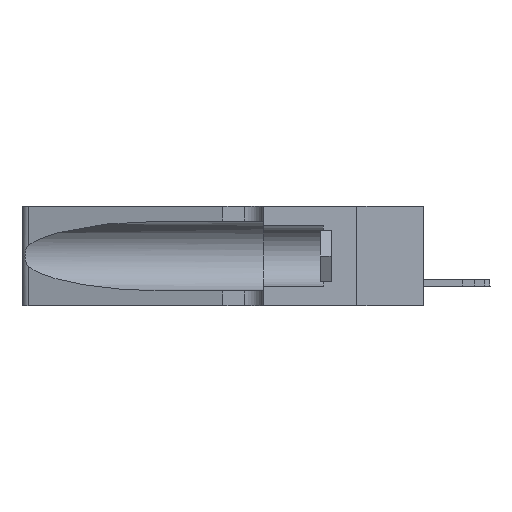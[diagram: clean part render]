
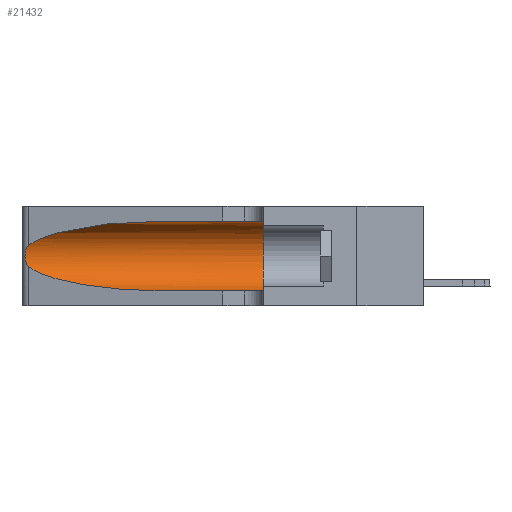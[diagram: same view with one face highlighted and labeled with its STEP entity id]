
A CAD part, left-side view. The second image highlights one B-rep face of the part: STEP entity #21432.
In plain terms, the highlighted cylindrical face has radius 3.308 mm (diameter 6.617 mm), a partial arc.
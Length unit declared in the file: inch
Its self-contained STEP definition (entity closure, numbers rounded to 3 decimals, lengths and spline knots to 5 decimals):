
#696 = CARTESIAN_POINT ( 'NONE',  ( 0.25487, 1.22718, 0.22369 ) ) ;
#796 = CARTESIAN_POINT ( 'NONE',  ( 0.25487, 1.22718, 0.14631 ) ) ;
#932 = VERTEX_POINT ( 'NONE', #16767 ) ;
#1752 = CARTESIAN_POINT ( 'NONE',  ( 0.1305, 0.35, 0.05475 ) ) ;
#2565 = DIRECTION ( 'NONE',  ( 0., 0., 1. ) ) ;
#3207 = CYLINDRICAL_SURFACE ( 'NONE', #23544, 0.13025 ) ;
#4286 = EDGE_CURVE ( 'NONE', #932, #13764, #8159, .T. ) ;
#4900 = CARTESIAN_POINT ( 'NONE',  ( 0.18966, 0.96281, 0.31525 ) ) ;
#5783 = CARTESIAN_POINT ( 'NONE',  ( 0.25787, 1.23484, 0.2124 ) ) ;
#5935 = EDGE_LOOP ( 'NONE', ( #15192, #30540, #15027, #8940, #6265, #22174 ) ) ;
#5982 = FACE_OUTER_BOUND ( 'NONE', #5935, .T. ) ;
#6265 = ORIENTED_EDGE ( 'NONE', *, *, #31190, .F. ) ;
#6501 = VERTEX_POINT ( 'NONE', #12126 ) ;
#7694 = CARTESIAN_POINT ( 'NONE',  ( 0.1305, 0.35, 0.185 ) ) ;
#7905 = DIRECTION ( 'NONE',  ( 0., -1., 0. ) ) ;
#8117 = CARTESIAN_POINT ( 'NONE',  ( 0.25639, 1.23184, 0.21858 ) ) ;
#8159 = LINE ( 'NONE', #20817, #13401 ) ;
#8224 = CARTESIAN_POINT ( 'NONE',  ( 0.18966, 0.96281, 0.05475 ) ) ;
#8459 = CARTESIAN_POINT ( 'NONE',  ( 0.2373, 1.15595, 0.08982 ) ) ;
#8463 = VERTEX_POINT ( 'NONE', #29225 ) ;
#8706 = CARTESIAN_POINT ( 'NONE',  ( 0.25639, 1.23186, 0.15144 ) ) ;
#8710 = EDGE_CURVE ( 'NONE', #8463, #6501, #29080, .T. ) ;
#8823 = CARTESIAN_POINT ( 'NONE',  ( 0.25555, 1.22993, 0.14849 ) ) ;
#8940 = ORIENTED_EDGE ( 'NONE', *, *, #4286, .T. ) ;
#9414 = DIRECTION ( 'NONE',  ( 0., -1., 0. ) ) ;
#10701 = DIRECTION ( 'NONE',  ( 0., 1., 0. ) ) ;
#11767 = CARTESIAN_POINT ( 'NONE',  ( 0.25856, 1.23593, 0.16098 ) ) ;
#11791 = VERTEX_POINT ( 'NONE', #26903 ) ;
#12126 = CARTESIAN_POINT ( 'NONE',  ( 0.25487, 1.22718, 0.22369 ) ) ;
#12245 = CARTESIAN_POINT ( 'NONE',  ( 0.25487, 1.22718, 0.14631 ) ) ;
#13401 = VECTOR ( 'NONE', #7905, 39.37008 ) ;
#13653 = CARTESIAN_POINT ( 'NONE',  ( 0.1305, 0.72297, 0.05475 ) ) ;
#13764 = VERTEX_POINT ( 'NONE', #1752 ) ;
#13896 = CARTESIAN_POINT ( 'NONE',  ( 0.25789, 1.23486, 0.15765 ) ) ;
#14348 = CARTESIAN_POINT ( 'NONE',  ( 0.26017, 1.23833, 0.17102 ) ) ;
#14768 = B_SPLINE_CURVE_WITH_KNOTS ( 'NONE', 3,
 ( #696, #26344, #8117, #5783, #23698, #26238, #31158, #29419, #14348, #11767, #13896, #8706, #8823, #29637 ),
 .UNSPECIFIED., .F., .F.,
 ( 4, 2, 2, 2, 2, 2, 4 ),
 ( 0., 0.00027, 0.00053, 0.00107, 0.0016, 0.00187, 0.00214 ),
 .UNSPECIFIED. ) ;
#15027 = ORIENTED_EDGE ( 'NONE', *, *, #16935, .T. ) ;
#15192 = ORIENTED_EDGE ( 'NONE', *, *, #8710, .T. ) ;
#16521 = LINE ( 'NONE', #27813, #30070 ) ;
#16767 = CARTESIAN_POINT ( 'NONE',  ( 0.1305, 0.72297, 0.05475 ) ) ;
#16935 = EDGE_CURVE ( 'NONE', #22032, #932, #18235, .T. ) ;
#17136 = CIRCLE ( 'NONE', #25724, 0.13025 ) ;
#18235 =( BOUNDED_CURVE ( )  B_SPLINE_CURVE ( 3, ( #796, #8459, #8224, #13653 ),
 .UNSPECIFIED., .F., .T. ) 
 B_SPLINE_CURVE_WITH_KNOTS ( ( 4, 4 ),
 ( 3.44316, 4.71239 ),
 .UNSPECIFIED. ) 
 CURVE ( )  GEOMETRIC_REPRESENTATION_ITEM ( )  RATIONAL_B_SPLINE_CURVE ( ( 1., 0.87, 0.87, 1. ) ) 
 REPRESENTATION_ITEM ( '' )  );
#19198 = CARTESIAN_POINT ( 'NONE',  ( 0.1305, 1.61858, 0.185 ) ) ;
#20817 = CARTESIAN_POINT ( 'NONE',  ( 0.1305, 1.61858, 0.05475 ) ) ;
#20926 = EDGE_CURVE ( 'NONE', #8463, #11791, #16521, .T. ) ;
#21432 = ADVANCED_FACE ( 'NONE', ( #5982 ), #3207, .F. ) ;
#22032 = VERTEX_POINT ( 'NONE', #12245 ) ;
#22174 = ORIENTED_EDGE ( 'NONE', *, *, #20926, .F. ) ;
#22838 = DIRECTION ( 'NONE',  ( 0., -1., 0. ) ) ;
#23544 = AXIS2_PLACEMENT_3D ( 'NONE', #19198, #9414, #27592 ) ;
#23698 = CARTESIAN_POINT ( 'NONE',  ( 0.25854, 1.2359, 0.20912 ) ) ;
#25724 = AXIS2_PLACEMENT_3D ( 'NONE', #7694, #10701, #2565 ) ;
#25805 = EDGE_CURVE ( 'NONE', #6501, #22032, #14768, .T. ) ;
#26238 = CARTESIAN_POINT ( 'NONE',  ( 0.26018, 1.23835, 0.19895 ) ) ;
#26344 = CARTESIAN_POINT ( 'NONE',  ( 0.25555, 1.22994, 0.2215 ) ) ;
#26903 = CARTESIAN_POINT ( 'NONE',  ( 0.1305, 0.35, 0.31525 ) ) ;
#27592 = DIRECTION ( 'NONE',  ( 0., 0., -1. ) ) ;
#27813 = CARTESIAN_POINT ( 'NONE',  ( 0.1305, 1.61858, 0.31525 ) ) ;
#29080 =( BOUNDED_CURVE ( )  B_SPLINE_CURVE ( 3, ( #32199, #4900, #31707, #30947 ),
 .UNSPECIFIED., .F., .T. ) 
 B_SPLINE_CURVE_WITH_KNOTS ( ( 4, 4 ),
 ( 1.5708, 2.84003 ),
 .UNSPECIFIED. ) 
 CURVE ( )  GEOMETRIC_REPRESENTATION_ITEM ( )  RATIONAL_B_SPLINE_CURVE ( ( 1., 0.87, 0.87, 1. ) ) 
 REPRESENTATION_ITEM ( '' )  );
#29225 = CARTESIAN_POINT ( 'NONE',  ( 0.1305, 0.72297, 0.31525 ) ) ;
#29419 = CARTESIAN_POINT ( 'NONE',  ( 0.26075, 1.23896, 0.178 ) ) ;
#29637 = CARTESIAN_POINT ( 'NONE',  ( 0.25487, 1.22718, 0.14631 ) ) ;
#30070 = VECTOR ( 'NONE', #22838, 39.37008 ) ;
#30540 = ORIENTED_EDGE ( 'NONE', *, *, #25805, .T. ) ;
#30947 = CARTESIAN_POINT ( 'NONE',  ( 0.25487, 1.22718, 0.22369 ) ) ;
#31158 = CARTESIAN_POINT ( 'NONE',  ( 0.26075, 1.23896, 0.19203 ) ) ;
#31190 = EDGE_CURVE ( 'NONE', #11791, #13764, #17136, .T. ) ;
#31707 = CARTESIAN_POINT ( 'NONE',  ( 0.2373, 1.15595, 0.28018 ) ) ;
#32199 = CARTESIAN_POINT ( 'NONE',  ( 0.1305, 0.72297, 0.31525 ) ) ;
